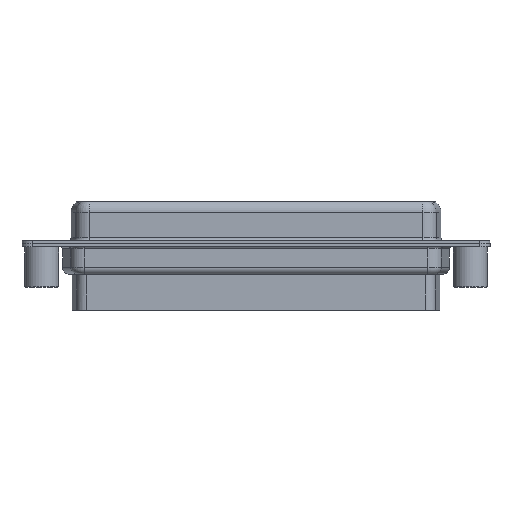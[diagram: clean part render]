
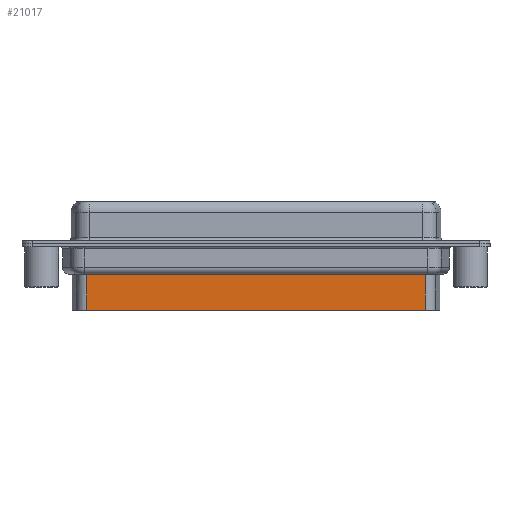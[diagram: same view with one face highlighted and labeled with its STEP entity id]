
A CAD part, front view. The second image highlights one B-rep face of the part: STEP entity #21017.
In plain terms, the highlighted planar face has unit normal (0, -1, 0).
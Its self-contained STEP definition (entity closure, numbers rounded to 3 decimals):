
#654 = VERTEX_POINT ( 'NONE', #9554 ) ;
#690 = CARTESIAN_POINT ( 'NONE',  ( 6.706, -3.5, -3.1 ) ) ;
#787 = CARTESIAN_POINT ( 'NONE',  ( 6.459, -3.5, -4.097 ) ) ;
#2084 = LINE ( 'NONE', #12118, #15734 ) ;
#2794 = LINE ( 'NONE', #3271, #19050 ) ;
#2851 = FACE_OUTER_BOUND ( 'NONE', #30927, .T. ) ;
#3168 = CARTESIAN_POINT ( 'NONE',  ( 56.794, -3.5, -4.097 ) ) ;
#3271 = CARTESIAN_POINT ( 'NONE',  ( 6.706, -3.5, -9.85 ) ) ;
#5576 = EDGE_CURVE ( 'NONE', #12311, #654, #13102, .T. ) ;
#5807 = ORIENTED_EDGE ( 'NONE', *, *, #5576, .T. ) ;
#9554 = CARTESIAN_POINT ( 'NONE',  ( 6.706, -3.5, -4.097 ) ) ;
#9782 = CARTESIAN_POINT ( 'NONE',  ( 6.706, -3.5, -3.1 ) ) ;
#10385 = AXIS2_PLACEMENT_3D ( 'NONE', #690, #20723, #31047 ) ;
#11303 = CARTESIAN_POINT ( 'NONE',  ( 6.706, -3.5, -9.85 ) ) ;
#11357 = ORIENTED_EDGE ( 'NONE', *, *, #32175, .F. ) ;
#12076 = DIRECTION ( 'NONE',  ( 0., 0., -1. ) ) ;
#12118 = CARTESIAN_POINT ( 'NONE',  ( 56.794, -3.5, -3.1 ) ) ;
#12311 = VERTEX_POINT ( 'NONE', #3168 ) ;
#12554 = ORIENTED_EDGE ( 'NONE', *, *, #27541, .T. ) ;
#12855 = PLANE ( 'NONE',  #10385 ) ;
#13102 = LINE ( 'NONE', #787, #18072 ) ;
#15734 = VECTOR ( 'NONE', #24397, 1000. ) ;
#18072 = VECTOR ( 'NONE', #30813, 1000. ) ;
#18074 = DIRECTION ( 'NONE',  ( -1., 0., 0. ) ) ;
#18580 = VERTEX_POINT ( 'NONE', #29149 ) ;
#18594 = ORIENTED_EDGE ( 'NONE', *, *, #23294, .F. ) ;
#19050 = VECTOR ( 'NONE', #18074, 1000. ) ;
#20723 = DIRECTION ( 'NONE',  ( 0., -1., 0. ) ) ;
#21017 = ADVANCED_FACE ( 'NONE', ( #2851 ), #12855, .T. ) ;
#23294 = EDGE_CURVE ( 'NONE', #12311, #18580, #2084, .T. ) ;
#24157 = VECTOR ( 'NONE', #12076, 1000. ) ;
#24397 = DIRECTION ( 'NONE',  ( 0., 0., -1. ) ) ;
#25000 = LINE ( 'NONE', #9782, #24157 ) ;
#27541 = EDGE_CURVE ( 'NONE', #654, #32275, #25000, .T. ) ;
#29149 = CARTESIAN_POINT ( 'NONE',  ( 56.794, -3.5, -9.85 ) ) ;
#30813 = DIRECTION ( 'NONE',  ( -1., 0., 0. ) ) ;
#30927 = EDGE_LOOP ( 'NONE', ( #18594, #5807, #12554, #11357 ) ) ;
#31047 = DIRECTION ( 'NONE',  ( 1., 0., 0. ) ) ;
#32175 = EDGE_CURVE ( 'NONE', #18580, #32275, #2794, .T. ) ;
#32275 = VERTEX_POINT ( 'NONE', #11303 ) ;
